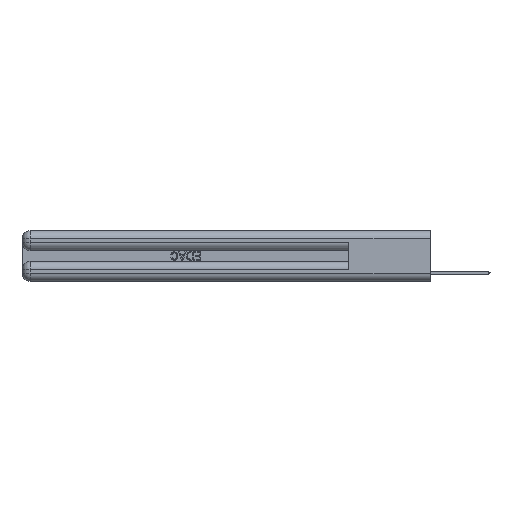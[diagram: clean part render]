
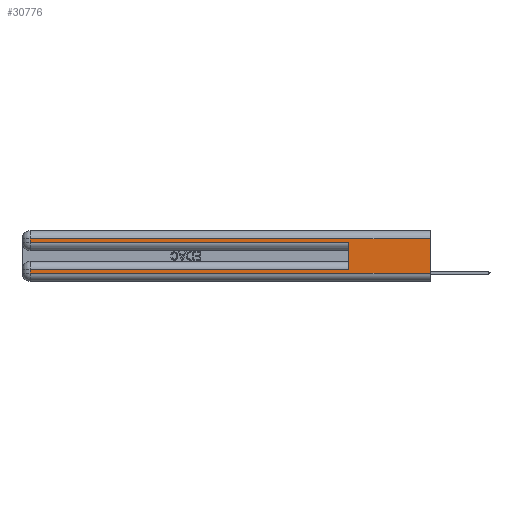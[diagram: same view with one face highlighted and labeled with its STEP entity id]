
A CAD part, left-side view. The second image highlights one B-rep face of the part: STEP entity #30776.
In plain terms, the highlighted planar face has unit normal (-1, 0, 0).
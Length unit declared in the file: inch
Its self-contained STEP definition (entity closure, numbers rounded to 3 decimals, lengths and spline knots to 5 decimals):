
#576 = DIRECTION ( 'NONE',  ( 0., 0., -1. ) ) ;
#634 = DIRECTION ( 'NONE',  ( 0., 1., 0. ) ) ;
#1108 = ORIENTED_EDGE ( 'NONE', *, *, #2338, .T. ) ;
#1150 = LINE ( 'NONE', #21959, #10530 ) ;
#1164 = DIRECTION ( 'NONE',  ( 0., -1., 0. ) ) ;
#1696 = VERTEX_POINT ( 'NONE', #29076 ) ;
#2076 = AXIS2_PLACEMENT_3D ( 'NONE', #25074, #8669, #10694 ) ;
#2338 = EDGE_CURVE ( 'NONE', #21187, #1696, #15669, .T. ) ;
#3467 = CARTESIAN_POINT ( 'NONE',  ( 0., 0., 0.31 ) ) ;
#4345 = CARTESIAN_POINT ( 'NONE',  ( 0., 2.94, 0.06 ) ) ;
#5113 = DIRECTION ( 'NONE',  ( 0., 1., 0. ) ) ;
#5511 = DIRECTION ( 'NONE',  ( 0., 0., -1. ) ) ;
#6499 = VERTEX_POINT ( 'NONE', #23925 ) ;
#6910 = VECTOR ( 'NONE', #5511, 39.37008 ) ;
#7536 = EDGE_CURVE ( 'NONE', #28559, #9999, #16982, .T. ) ;
#8669 = DIRECTION ( 'NONE',  ( 1., 0., 0. ) ) ;
#9006 = CARTESIAN_POINT ( 'NONE',  ( 0., 0., 0.06 ) ) ;
#9773 = VERTEX_POINT ( 'NONE', #4345 ) ;
#9799 = EDGE_CURVE ( 'NONE', #9773, #6499, #16437, .T. ) ;
#9999 = VERTEX_POINT ( 'NONE', #15573 ) ;
#10289 = EDGE_CURVE ( 'NONE', #9999, #9773, #1150, .T. ) ;
#10530 = VECTOR ( 'NONE', #576, 39.37008 ) ;
#10694 = DIRECTION ( 'NONE',  ( 0., 0., -1. ) ) ;
#11218 = VECTOR ( 'NONE', #1164, 39.37008 ) ;
#11533 = DIRECTION ( 'NONE',  ( 0., -1., 0. ) ) ;
#12142 = CARTESIAN_POINT ( 'NONE',  ( 0., 2.94, 0.31 ) ) ;
#13249 = LINE ( 'NONE', #24968, #21348 ) ;
#13290 = EDGE_CURVE ( 'NONE', #15416, #6499, #26320, .T. ) ;
#13709 = CARTESIAN_POINT ( 'NONE',  ( 0., 0.6, 0.085 ) ) ;
#13794 = EDGE_CURVE ( 'NONE', #21636, #21187, #13249, .T. ) ;
#14946 = EDGE_LOOP ( 'NONE', ( #30423, #20189, #16729, #1108, #29034, #28534, #24237, #25203 ) ) ;
#15416 = VERTEX_POINT ( 'NONE', #3467 ) ;
#15507 = DIRECTION ( 'NONE',  ( 0., 0., 1. ) ) ;
#15573 = CARTESIAN_POINT ( 'NONE',  ( 0., 2.94, 0.085 ) ) ;
#15669 = LINE ( 'NONE', #20205, #11218 ) ;
#15729 = VECTOR ( 'NONE', #11533, 39.37008 ) ;
#15775 = PLANE ( 'NONE',  #2076 ) ;
#16437 = LINE ( 'NONE', #9006, #15729 ) ;
#16729 = ORIENTED_EDGE ( 'NONE', *, *, #13794, .T. ) ;
#16982 = LINE ( 'NONE', #23753, #27362 ) ;
#17194 = CARTESIAN_POINT ( 'NONE',  ( 0., 0., 0.31 ) ) ;
#19219 = EDGE_CURVE ( 'NONE', #28559, #1696, #21409, .T. ) ;
#19535 = CARTESIAN_POINT ( 'NONE',  ( 0., 0., 0.37 ) ) ;
#20189 = ORIENTED_EDGE ( 'NONE', *, *, #25305, .T. ) ;
#20205 = CARTESIAN_POINT ( 'NONE',  ( 0., 0., 0.285 ) ) ;
#21187 = VERTEX_POINT ( 'NONE', #27094 ) ;
#21348 = VECTOR ( 'NONE', #25282, 39.37008 ) ;
#21409 = LINE ( 'NONE', #27299, #28480 ) ;
#21636 = VERTEX_POINT ( 'NONE', #12142 ) ;
#21959 = CARTESIAN_POINT ( 'NONE',  ( 0., 2.94, 0.37 ) ) ;
#22285 = LINE ( 'NONE', #17194, #25637 ) ;
#23753 = CARTESIAN_POINT ( 'NONE',  ( 0., 0., 0.085 ) ) ;
#23925 = CARTESIAN_POINT ( 'NONE',  ( 0., 0., 0.06 ) ) ;
#24237 = ORIENTED_EDGE ( 'NONE', *, *, #10289, .T. ) ;
#24615 = FACE_OUTER_BOUND ( 'NONE', #14946, .T. ) ;
#24968 = CARTESIAN_POINT ( 'NONE',  ( 0., 2.94, 0.37 ) ) ;
#25074 = CARTESIAN_POINT ( 'NONE',  ( 0., 0., 0.37 ) ) ;
#25203 = ORIENTED_EDGE ( 'NONE', *, *, #9799, .T. ) ;
#25282 = DIRECTION ( 'NONE',  ( 0., 0., -1. ) ) ;
#25305 = EDGE_CURVE ( 'NONE', #15416, #21636, #22285, .T. ) ;
#25637 = VECTOR ( 'NONE', #634, 39.37008 ) ;
#26320 = LINE ( 'NONE', #19535, #6910 ) ;
#27094 = CARTESIAN_POINT ( 'NONE',  ( 0., 2.94, 0.285 ) ) ;
#27299 = CARTESIAN_POINT ( 'NONE',  ( 0., 0.6, 0.145 ) ) ;
#27362 = VECTOR ( 'NONE', #5113, 39.37008 ) ;
#28480 = VECTOR ( 'NONE', #15507, 39.37008 ) ;
#28534 = ORIENTED_EDGE ( 'NONE', *, *, #7536, .T. ) ;
#28559 = VERTEX_POINT ( 'NONE', #13709 ) ;
#29034 = ORIENTED_EDGE ( 'NONE', *, *, #19219, .F. ) ;
#29076 = CARTESIAN_POINT ( 'NONE',  ( 0., 0.6, 0.285 ) ) ;
#30423 = ORIENTED_EDGE ( 'NONE', *, *, #13290, .F. ) ;
#30776 = ADVANCED_FACE ( 'NONE', ( #24615 ), #15775, .F. ) ;
